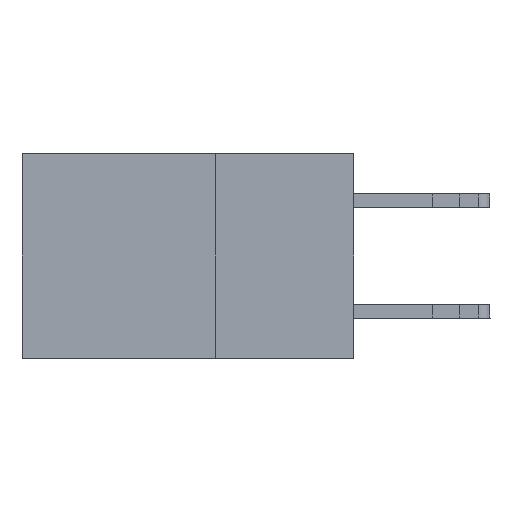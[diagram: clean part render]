
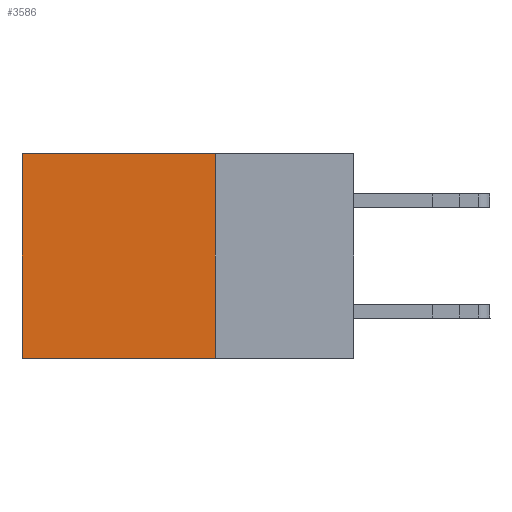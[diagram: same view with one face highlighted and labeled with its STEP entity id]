
A CAD part, left-side view. The second image highlights one B-rep face of the part: STEP entity #3586.
In plain terms, the highlighted planar face has unit normal (-1, 0, 0).
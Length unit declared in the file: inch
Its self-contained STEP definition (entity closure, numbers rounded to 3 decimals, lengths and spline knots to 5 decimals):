
#912 = EDGE_CURVE ( 'NONE', #30766, #15490, #31612, .T. ) ;
#3586 = ADVANCED_FACE ( 'NONE', ( #18240 ), #23422, .F. ) ;
#4290 = DIRECTION ( 'NONE',  ( 1., 0., 0. ) ) ;
#4545 = CARTESIAN_POINT ( 'NONE',  ( 0.2875, 0.25, -0.37 ) ) ;
#5386 = ORIENTED_EDGE ( 'NONE', *, *, #34735, .F. ) ;
#6746 = VECTOR ( 'NONE', #22730, 39.37008 ) ;
#7191 = EDGE_LOOP ( 'NONE', ( #33932, #5386, #28592, #28881 ) ) ;
#7530 = CARTESIAN_POINT ( 'NONE',  ( 0.2875, 0.25, 0. ) ) ;
#7716 = DIRECTION ( 'NONE',  ( 0., 1., 0. ) ) ;
#11811 = EDGE_CURVE ( 'NONE', #33745, #30766, #32181, .T. ) ;
#15490 = VERTEX_POINT ( 'NONE', #32267 ) ;
#16174 = VECTOR ( 'NONE', #16712, 39.37008 ) ;
#16712 = DIRECTION ( 'NONE',  ( 0., 1., 0. ) ) ;
#17374 = CARTESIAN_POINT ( 'NONE',  ( 0.2875, 0.25, 0. ) ) ;
#18086 = CARTESIAN_POINT ( 'NONE',  ( 0.2875, 0.25, 0. ) ) ;
#18240 = FACE_OUTER_BOUND ( 'NONE', #7191, .T. ) ;
#19728 = LINE ( 'NONE', #30255, #16174 ) ;
#20598 = LINE ( 'NONE', #17374, #6746 ) ;
#22624 = VERTEX_POINT ( 'NONE', #4545 ) ;
#22730 = DIRECTION ( 'NONE',  ( 0., 0., -1. ) ) ;
#23422 = PLANE ( 'NONE',  #26884 ) ;
#24164 = CARTESIAN_POINT ( 'NONE',  ( 0.2875, 0.25, 0. ) ) ;
#26826 = DIRECTION ( 'NONE',  ( 0., 0., -1. ) ) ;
#26884 = AXIS2_PLACEMENT_3D ( 'NONE', #7530, #4290, #29144 ) ;
#27420 = VECTOR ( 'NONE', #26826, 39.37008 ) ;
#27707 = EDGE_CURVE ( 'NONE', #33745, #22624, #20598, .T. ) ;
#28592 = ORIENTED_EDGE ( 'NONE', *, *, #27707, .F. ) ;
#28881 = ORIENTED_EDGE ( 'NONE', *, *, #11811, .T. ) ;
#28960 = CARTESIAN_POINT ( 'NONE',  ( 0.2875, 0.6, 0. ) ) ;
#29144 = DIRECTION ( 'NONE',  ( 0., 0., -1. ) ) ;
#30255 = CARTESIAN_POINT ( 'NONE',  ( 0.2875, 0.25, -0.37 ) ) ;
#30766 = VERTEX_POINT ( 'NONE', #33454 ) ;
#31612 = LINE ( 'NONE', #28960, #27420 ) ;
#32181 = LINE ( 'NONE', #24164, #32860 ) ;
#32267 = CARTESIAN_POINT ( 'NONE',  ( 0.2875, 0.6, -0.37 ) ) ;
#32860 = VECTOR ( 'NONE', #7716, 39.37008 ) ;
#33454 = CARTESIAN_POINT ( 'NONE',  ( 0.2875, 0.6, 0. ) ) ;
#33745 = VERTEX_POINT ( 'NONE', #18086 ) ;
#33932 = ORIENTED_EDGE ( 'NONE', *, *, #912, .T. ) ;
#34735 = EDGE_CURVE ( 'NONE', #22624, #15490, #19728, .T. ) ;
